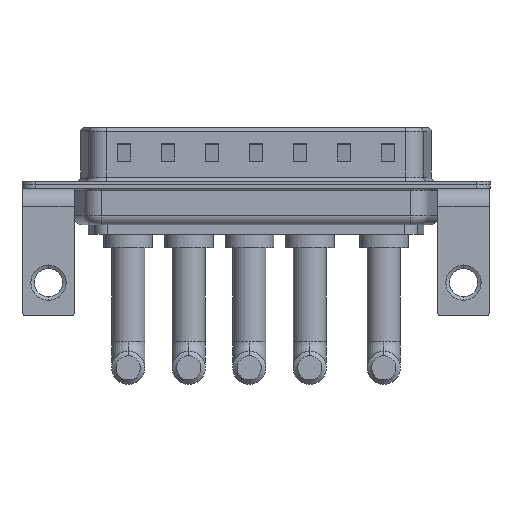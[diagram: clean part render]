
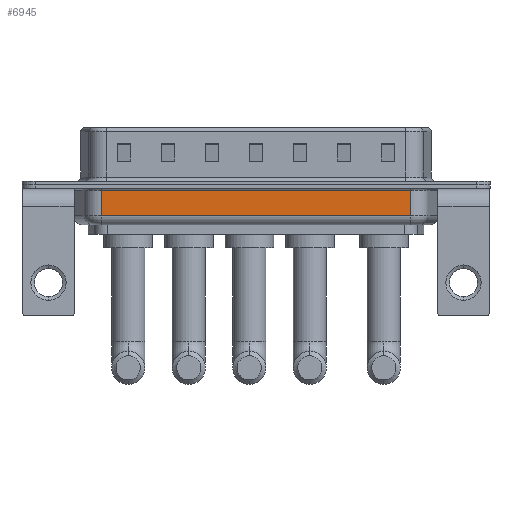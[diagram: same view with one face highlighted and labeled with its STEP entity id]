
A CAD part, front view. The second image highlights one B-rep face of the part: STEP entity #6945.
In plain terms, the highlighted planar face has unit normal (0, -1, 0).
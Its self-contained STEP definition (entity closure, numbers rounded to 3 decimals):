
#282 = LINE ( 'NONE', #5041, #12738 ) ;
#626 = EDGE_LOOP ( 'NONE', ( #8641, #2838, #3605, #2661 ) ) ;
#1139 = CARTESIAN_POINT ( 'NONE',  ( 6.006, -5.35, -3.5 ) ) ;
#2052 = CARTESIAN_POINT ( 'NONE',  ( 41.044, -5.35, -0.65 ) ) ;
#2661 = ORIENTED_EDGE ( 'NONE', *, *, #12141, .T. ) ;
#2838 = ORIENTED_EDGE ( 'NONE', *, *, #9121, .T. ) ;
#3002 = DIRECTION ( 'NONE',  ( 0., 0., 1. ) ) ;
#3106 = CARTESIAN_POINT ( 'NONE',  ( 6.006, -5.35, -3.5 ) ) ;
#3560 = VECTOR ( 'NONE', #8389, 1000. ) ;
#3605 = ORIENTED_EDGE ( 'NONE', *, *, #7997, .T. ) ;
#4445 = LINE ( 'NONE', #1139, #4554 ) ;
#4554 = VECTOR ( 'NONE', #14954, 1000. ) ;
#4589 = FACE_OUTER_BOUND ( 'NONE', #626, .T. ) ;
#4718 = CARTESIAN_POINT ( 'NONE',  ( 41.044, -5.35, -3.5 ) ) ;
#5041 = CARTESIAN_POINT ( 'NONE',  ( 6.006, -5.35, -0.65 ) ) ;
#5400 = CARTESIAN_POINT ( 'NONE',  ( 6.006, -5.35, -0.65 ) ) ;
#5524 = AXIS2_PLACEMENT_3D ( 'NONE', #5972, #9266, #10672 ) ;
#5597 = LINE ( 'NONE', #11369, #7614 ) ;
#5972 = CARTESIAN_POINT ( 'NONE',  ( 6.006, -5.35, -4.5 ) ) ;
#6174 = VERTEX_POINT ( 'NONE', #4718 ) ;
#6945 = ADVANCED_FACE ( 'NONE', ( #4589 ), #12661, .F. ) ;
#7614 = VECTOR ( 'NONE', #3002, 1000. ) ;
#7997 = EDGE_CURVE ( 'NONE', #6174, #14049, #10705, .T. ) ;
#8389 = DIRECTION ( 'NONE',  ( 0., 0., 1. ) ) ;
#8641 = ORIENTED_EDGE ( 'NONE', *, *, #13465, .F. ) ;
#9121 = EDGE_CURVE ( 'NONE', #11875, #6174, #4445, .T. ) ;
#9266 = DIRECTION ( 'NONE',  ( 0., 1., 0. ) ) ;
#10032 = VERTEX_POINT ( 'NONE', #5400 ) ;
#10672 = DIRECTION ( 'NONE',  ( 0., 0., 1. ) ) ;
#10705 = LINE ( 'NONE', #11843, #3560 ) ;
#11369 = CARTESIAN_POINT ( 'NONE',  ( 6.006, -5.35, -4.5 ) ) ;
#11843 = CARTESIAN_POINT ( 'NONE',  ( 41.044, -5.35, -4.5 ) ) ;
#11875 = VERTEX_POINT ( 'NONE', #3106 ) ;
#12141 = EDGE_CURVE ( 'NONE', #14049, #10032, #282, .T. ) ;
#12661 = PLANE ( 'NONE',  #5524 ) ;
#12738 = VECTOR ( 'NONE', #13028, 1000. ) ;
#13028 = DIRECTION ( 'NONE',  ( -1., 0., 0. ) ) ;
#13465 = EDGE_CURVE ( 'NONE', #11875, #10032, #5597, .T. ) ;
#14049 = VERTEX_POINT ( 'NONE', #2052 ) ;
#14954 = DIRECTION ( 'NONE',  ( 1., 0., 0. ) ) ;
